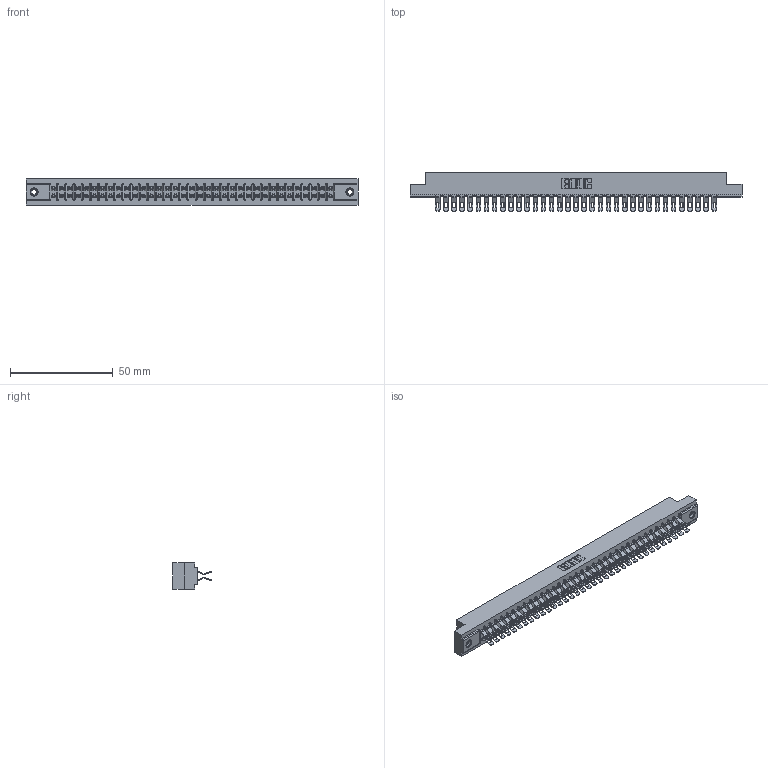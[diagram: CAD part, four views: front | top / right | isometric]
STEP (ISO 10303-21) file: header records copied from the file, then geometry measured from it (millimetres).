
FILE_DESCRIPTION (( 'STEP AP203' ), '1' );
FILE_NAME ('357-070-455-208.STEP', '2020-10-04T21:33:10', ( '' ), ( '' ), 'SwSTEP 2.0', 'SolidWorks 2020', '' );
FILE_SCHEMA (( 'CONFIG_CONTROL_DESIGN' ));
Length unit declared in the file: inch
Products named in the file (4): 345-250-001_345-250-003-102; 307-290-001_555; 357-070-455-208; 307 Part_.156 Dia Mounting Holes
Assembly tree (73 placements, depth 2):
  357-070-455-208
    307 Part_.156 Dia Mounting Holes
    307-290-001_555  x70
    345-250-001_345-250-003-102  x2
Bounding box: 161.7 x 18.75 x 12.7 mm (x, y, z)
Volume: 17346.9 mm3; surface area: 22261.9 mm2
Topology: 73 solids, 73 shells, 4484 faces, 13129 edges, 8554 vertices
Faces by surface type: plane 2482, cylinder 1914, sphere 72, cone 12, torus 4
Entity records: 33710 total; most frequent: CARTESIAN_POINT 5506, ORIENTED_EDGE 5452, DIRECTION 5412, EDGE_CURVE 2726, VECTOR 2076, LINE 2076, VERTEX_POINT 1762, AXIS2_PLACEMENT_3D 1668
